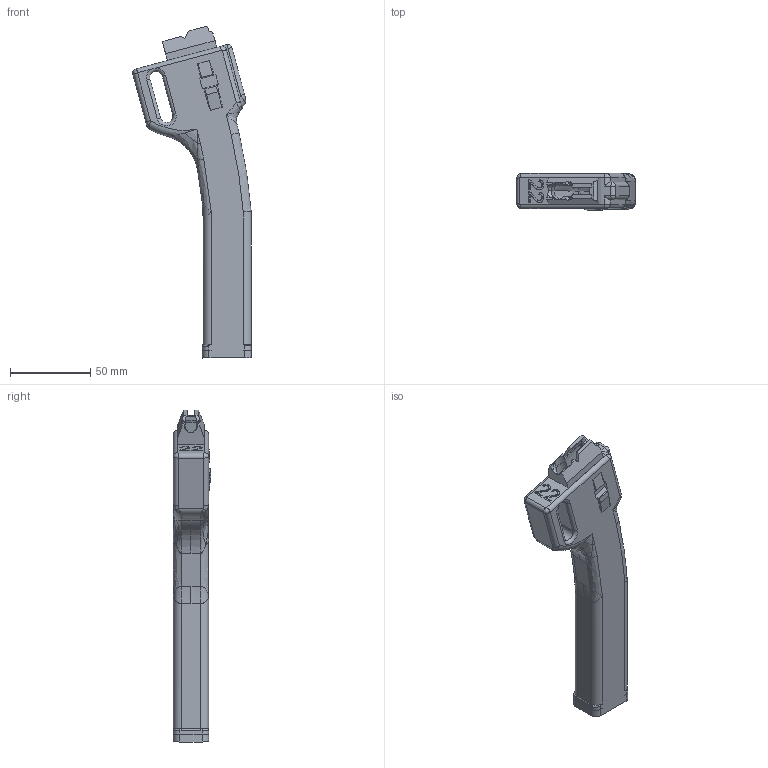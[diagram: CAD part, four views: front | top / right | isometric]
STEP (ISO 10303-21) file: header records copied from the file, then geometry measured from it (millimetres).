
FILE_DESCRIPTION(/* description */ (''),/* implementation_level */ '2;1');
FILE_NAME(/* name */ 'ar1522magslim.step',/* time_stamp */ '2021-10-16T18:40:19-04:00',/* author */ (''),/* organization */ (''),/* preprocessor_version */ 'ST-DEVELOPER v18.1',/* originating_system */ 'Autodesk Translation Framework v10.10.0.1391',/* authorisation */ '');
FILE_SCHEMA (('AUTOMOTIVE_DESIGN { 1 0 10303 214 3 1 1 }'));
Length unit declared in the file: millimetre
Products named in the file (3): ar mp5 mag; mp5 v16; BodyCombined-new (1)
Assembly tree (2 placements, depth 3):
  ar mp5 mag
    mp5 v16
      BodyCombined-new (1)
Bounding box: 73.98 x 23.32 x 207.37 mm (x, y, z)
Volume: 110170.7 mm3; surface area: 40159.2 mm2
Topology: 1 solids, 1 shells, 371 faces, 1007 edges, 619 vertices
Faces by surface type: bspline 182, plane 107, cylinder 70, torus 10, sphere 2
Entity records: 17928 total; most frequent: CARTESIAN_POINT 9763, ORIENTED_EDGE 1980, DIRECTION 1231, EDGE_CURVE 990, VERTEX_POINT 619, AXIS2_PLACEMENT_3D 434, B_SPLINE_CURVE_WITH_KNOTS 387, EDGE_LOOP 377
